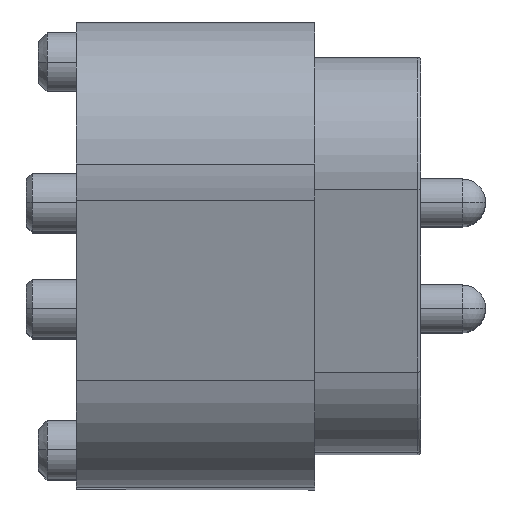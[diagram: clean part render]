
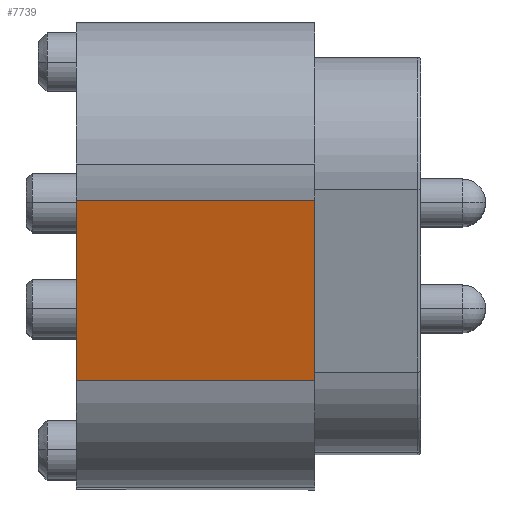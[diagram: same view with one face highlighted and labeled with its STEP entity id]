
A CAD part, top view. The second image highlights one B-rep face of the part: STEP entity #7739.
In plain terms, the highlighted planar face has unit normal (0, -0.247, 0.969).
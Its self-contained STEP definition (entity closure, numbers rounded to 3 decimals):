
#186 = VECTOR ( 'NONE', #6842, 1000. ) ;
#364 = ORIENTED_EDGE ( 'NONE', *, *, #5390, .T. ) ;
#387 = DIRECTION ( 'NONE',  ( 0., 0.969, 0.247 ) ) ;
#540 = LINE ( 'NONE', #3367, #7312 ) ;
#953 = EDGE_CURVE ( 'NONE', #2683, #3722, #540, .T. ) ;
#976 = VERTEX_POINT ( 'NONE', #6277 ) ;
#1124 = LINE ( 'NONE', #3963, #186 ) ;
#1499 = ORIENTED_EDGE ( 'NONE', *, *, #4071, .F. ) ;
#1734 = DIRECTION ( 'NONE',  ( -1., 0., 0. ) ) ;
#2104 = CARTESIAN_POINT ( 'NONE',  ( -122.073, -9.678, 14.748 ) ) ;
#2428 = PLANE ( 'NONE',  #3461 ) ;
#2683 = VERTEX_POINT ( 'NONE', #3357 ) ;
#3152 = VECTOR ( 'NONE', #4970, 1000. ) ;
#3357 = CARTESIAN_POINT ( 'NONE',  ( -118.023, -6.616, 15.529 ) ) ;
#3367 = CARTESIAN_POINT ( 'NONE',  ( -118.023, -6.616, 15.529 ) ) ;
#3461 = AXIS2_PLACEMENT_3D ( 'NONE', #5300, #8140, #1734 ) ;
#3722 = VERTEX_POINT ( 'NONE', #6134 ) ;
#3916 = LINE ( 'NONE', #6798, #8022 ) ;
#3963 = CARTESIAN_POINT ( 'NONE',  ( -118.023, -6.616, 15.529 ) ) ;
#4071 = EDGE_CURVE ( 'NONE', #6726, #976, #3916, .T. ) ;
#4970 = DIRECTION ( 'NONE',  ( 1., 0., 0. ) ) ;
#5101 = ORIENTED_EDGE ( 'NONE', *, *, #5570, .T. ) ;
#5300 = CARTESIAN_POINT ( 'NONE',  ( -120.048, -8.147, 15.139 ) ) ;
#5390 = EDGE_CURVE ( 'NONE', #2683, #976, #1124, .T. ) ;
#5570 = EDGE_CURVE ( 'NONE', #6726, #3722, #8507, .T. ) ;
#6134 = CARTESIAN_POINT ( 'NONE',  ( -118.023, -9.678, 14.748 ) ) ;
#6232 = DIRECTION ( 'NONE',  ( 0., -0.969, -0.247 ) ) ;
#6277 = CARTESIAN_POINT ( 'NONE',  ( -122.073, -6.616, 15.529 ) ) ;
#6309 = EDGE_LOOP ( 'NONE', ( #1499, #5101, #7644, #364 ) ) ;
#6726 = VERTEX_POINT ( 'NONE', #7757 ) ;
#6798 = CARTESIAN_POINT ( 'NONE',  ( -122.073, -6.835, 15.473 ) ) ;
#6842 = DIRECTION ( 'NONE',  ( -1., 0., 0. ) ) ;
#7312 = VECTOR ( 'NONE', #6232, 1000. ) ;
#7644 = ORIENTED_EDGE ( 'NONE', *, *, #953, .F. ) ;
#7739 = ADVANCED_FACE ( 'NONE', ( #8833 ), #2428, .T. ) ;
#7757 = CARTESIAN_POINT ( 'NONE',  ( -122.073, -9.678, 14.748 ) ) ;
#8022 = VECTOR ( 'NONE', #387, 1000. ) ;
#8140 = DIRECTION ( 'NONE',  ( 0., -0.247, 0.969 ) ) ;
#8507 = LINE ( 'NONE', #2104, #3152 ) ;
#8833 = FACE_OUTER_BOUND ( 'NONE', #6309, .T. ) ;
